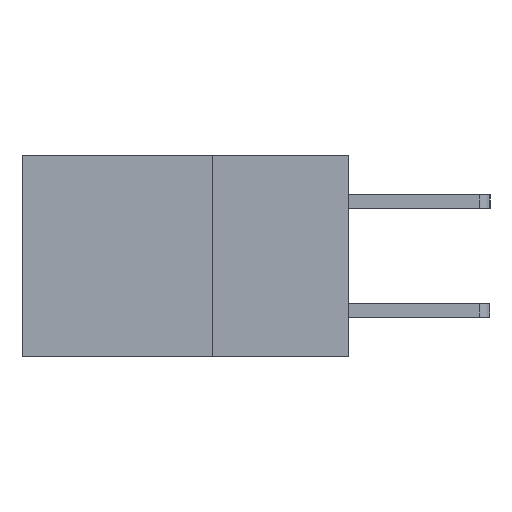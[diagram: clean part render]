
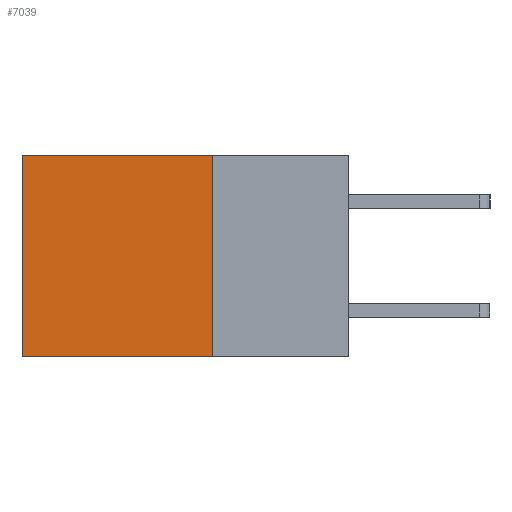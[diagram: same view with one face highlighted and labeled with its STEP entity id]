
A CAD part, left-side view. The second image highlights one B-rep face of the part: STEP entity #7039.
In plain terms, the highlighted planar face has unit normal (-1, 0, 0).
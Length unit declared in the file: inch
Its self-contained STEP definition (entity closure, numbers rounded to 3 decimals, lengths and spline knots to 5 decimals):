
#116 = CARTESIAN_POINT ( 'NONE',  ( 0.298, 0.25, 0. ) ) ;
#233 = AXIS2_PLACEMENT_3D ( 'NONE', #7461, #7505, #7258 ) ;
#243 = DIRECTION ( 'NONE',  ( 0., 1., 0. ) ) ;
#931 = ORIENTED_EDGE ( 'NONE', *, *, #3673, .T. ) ;
#1561 = VECTOR ( 'NONE', #1671, 39.37008 ) ;
#1671 = DIRECTION ( 'NONE',  ( 0., 0., -1. ) ) ;
#2258 = ORIENTED_EDGE ( 'NONE', *, *, #4975, .F. ) ;
#3234 = VERTEX_POINT ( 'NONE', #4005 ) ;
#3559 = VERTEX_POINT ( 'NONE', #5059 ) ;
#3673 = EDGE_CURVE ( 'NONE', #9609, #3559, #4429, .T. ) ;
#3760 = ORIENTED_EDGE ( 'NONE', *, *, #4832, .F. ) ;
#4005 = CARTESIAN_POINT ( 'NONE',  ( 0.298, 0.25, -0.37 ) ) ;
#4018 = CARTESIAN_POINT ( 'NONE',  ( 0.298, 0.6, 0. ) ) ;
#4079 = EDGE_CURVE ( 'NONE', #3559, #5494, #10234, .T. ) ;
#4257 = VECTOR ( 'NONE', #5819, 39.37008 ) ;
#4429 = LINE ( 'NONE', #8163, #8330 ) ;
#4438 = ORIENTED_EDGE ( 'NONE', *, *, #4079, .T. ) ;
#4454 = EDGE_LOOP ( 'NONE', ( #4438, #2258, #3760, #931 ) ) ;
#4585 = CARTESIAN_POINT ( 'NONE',  ( 0.298, 0.25, 0. ) ) ;
#4832 = EDGE_CURVE ( 'NONE', #9609, #3234, #6165, .T. ) ;
#4975 = EDGE_CURVE ( 'NONE', #3234, #5494, #8646, .T. ) ;
#5059 = CARTESIAN_POINT ( 'NONE',  ( 0.298, 0.6, 0. ) ) ;
#5494 = VERTEX_POINT ( 'NONE', #6471 ) ;
#5667 = CARTESIAN_POINT ( 'NONE',  ( 0.298, 0.25, -0.37 ) ) ;
#5819 = DIRECTION ( 'NONE',  ( 0., 1., 0. ) ) ;
#5901 = VECTOR ( 'NONE', #10075, 39.37008 ) ;
#6165 = LINE ( 'NONE', #4585, #5901 ) ;
#6471 = CARTESIAN_POINT ( 'NONE',  ( 0.298, 0.6, -0.37 ) ) ;
#7039 = ADVANCED_FACE ( 'NONE', ( #9513 ), #10232, .F. ) ;
#7258 = DIRECTION ( 'NONE',  ( 0., 0., -1. ) ) ;
#7461 = CARTESIAN_POINT ( 'NONE',  ( 0.298, 0.25, 0. ) ) ;
#7505 = DIRECTION ( 'NONE',  ( 1., 0., 0. ) ) ;
#8163 = CARTESIAN_POINT ( 'NONE',  ( 0.298, 0.25, 0. ) ) ;
#8330 = VECTOR ( 'NONE', #243, 39.37008 ) ;
#8646 = LINE ( 'NONE', #5667, #4257 ) ;
#9513 = FACE_OUTER_BOUND ( 'NONE', #4454, .T. ) ;
#9609 = VERTEX_POINT ( 'NONE', #116 ) ;
#10075 = DIRECTION ( 'NONE',  ( 0., 0., -1. ) ) ;
#10232 = PLANE ( 'NONE',  #233 ) ;
#10234 = LINE ( 'NONE', #4018, #1561 ) ;
